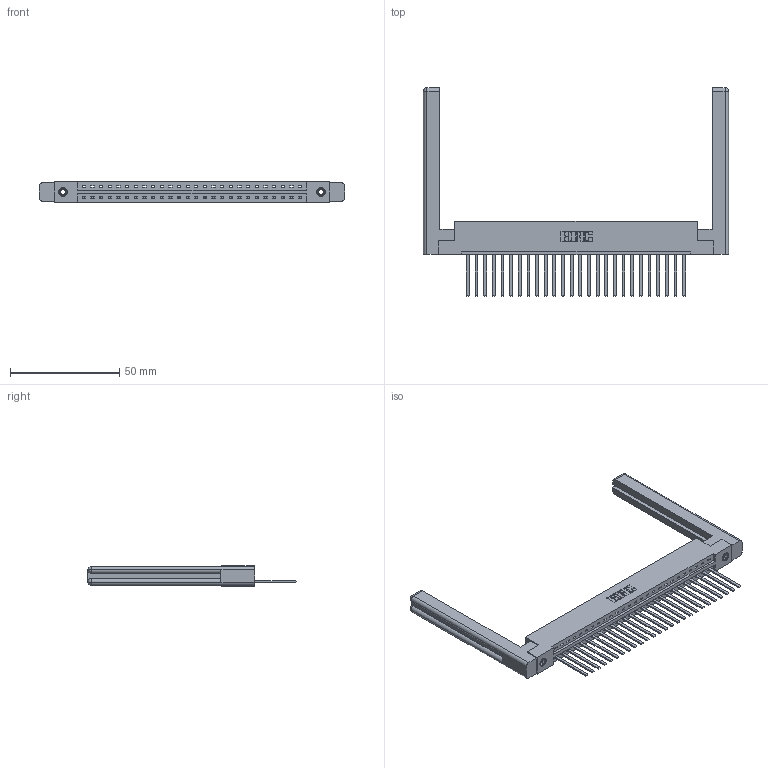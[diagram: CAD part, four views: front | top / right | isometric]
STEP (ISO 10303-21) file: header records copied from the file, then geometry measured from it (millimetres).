
FILE_DESCRIPTION (( 'STEP AP203' ), '1' );
FILE_NAME ('387-026-544-158.STEP', '2019-10-03T13:04:53', ( '' ), ( '' ), 'SwSTEP 2.0', 'SolidWorks 2016', '' );
FILE_SCHEMA (( 'CONFIG_CONTROL_DESIGN' ));
Length unit declared in the file: inch
Products named in the file (5): 345-292-001_345-293-144; 337 Part_Flush Mounting Lugs - 0.156 Dia-TI; 307-220-058; 345-250-001_345-250-001-102; 387-026-544-158
Assembly tree (31 placements, depth 2):
  387-026-544-158
    337 Part_Flush Mounting Lugs - 0.156 Dia-TI
    345-292-001_345-293-144  x26
    345-250-001_345-250-001-102  x2
    307-220-058  x2
Bounding box: 139.65 x 95.38 x 9.4 mm (x, y, z)
Volume: 21777.2 mm3; surface area: 21217.3 mm2
Topology: 31 solids, 31 shells, 1712 faces, 5085 edges, 3342 vertices
Faces by surface type: plane 1246, cylinder 442, cone 12, torus 12
Entity records: 23846 total; most frequent: CARTESIAN_POINT 4151, ORIENTED_EDGE 4052, DIRECTION 3542, EDGE_CURVE 2026, VECTOR 1854, LINE 1854, VERTEX_POINT 1342, AXIS2_PLACEMENT_3D 844
